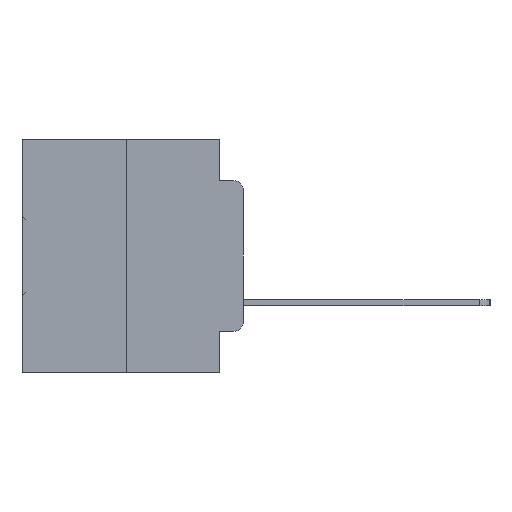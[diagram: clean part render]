
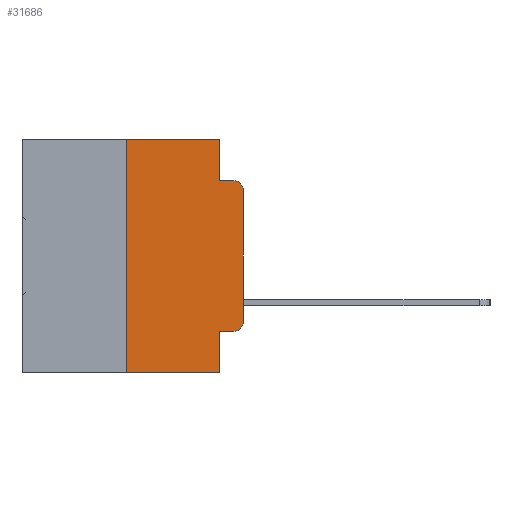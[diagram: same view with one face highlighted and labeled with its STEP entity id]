
A CAD part, left-side view. The second image highlights one B-rep face of the part: STEP entity #31686.
In plain terms, the highlighted planar face has unit normal (-1, 0, 0).
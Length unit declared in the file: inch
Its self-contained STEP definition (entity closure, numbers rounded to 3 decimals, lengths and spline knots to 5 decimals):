
#18 = LINE ( 'NONE', #4390, #19314 ) ;
#545 = CARTESIAN_POINT ( 'NONE',  ( 0., 0.051, -0.0885 ) ) ;
#846 = CARTESIAN_POINT ( 'NONE',  ( 0., 0.02, -0.0885 ) ) ;
#1336 = DIRECTION ( 'NONE',  ( -1., 0., 0. ) ) ;
#1484 = DIRECTION ( 'NONE',  ( 1., 0., 0. ) ) ;
#1604 = VERTEX_POINT ( 'NONE', #846 ) ;
#2535 = VERTEX_POINT ( 'NONE', #27322 ) ;
#2682 = CARTESIAN_POINT ( 'NONE',  ( 0., 0.02, -0.4115 ) ) ;
#3619 = VECTOR ( 'NONE', #10777, 39.37008 ) ;
#3819 = VERTEX_POINT ( 'NONE', #11487 ) ;
#3992 = EDGE_CURVE ( 'NONE', #10135, #1604, #17710, .T. ) ;
#4390 = CARTESIAN_POINT ( 'NONE',  ( 0., 0., 0. ) ) ;
#5689 = EDGE_CURVE ( 'NONE', #13016, #10135, #18, .T. ) ;
#5801 = DIRECTION ( 'NONE',  ( 0., -1., 0. ) ) ;
#5893 = EDGE_CURVE ( 'NONE', #17579, #13016, #7960, .T. ) ;
#6209 = VECTOR ( 'NONE', #22837, 39.37008 ) ;
#6605 = PLANE ( 'NONE',  #25079 ) ;
#7326 = CARTESIAN_POINT ( 'NONE',  ( 0., 0.473, -0.5 ) ) ;
#7960 = CIRCLE ( 'NONE', #10447, 0.02 ) ;
#8567 = EDGE_CURVE ( 'NONE', #21076, #2535, #12137, .T. ) ;
#9147 = DIRECTION ( 'NONE',  ( 0., 0., -1. ) ) ;
#9686 = LINE ( 'NONE', #28645, #22081 ) ;
#10097 = VECTOR ( 'NONE', #10678, 39.37008 ) ;
#10131 = ORIENTED_EDGE ( 'NONE', *, *, #5893, .T. ) ;
#10135 = VERTEX_POINT ( 'NONE', #13831 ) ;
#10249 = DIRECTION ( 'NONE',  ( -1., 0., 0. ) ) ;
#10447 = AXIS2_PLACEMENT_3D ( 'NONE', #24980, #10249, #27399 ) ;
#10678 = DIRECTION ( 'NONE',  ( 0., 0., -1. ) ) ;
#10777 = DIRECTION ( 'NONE',  ( 0., -1., 0. ) ) ;
#10806 = CARTESIAN_POINT ( 'NONE',  ( 0., 0.051, -0.4115 ) ) ;
#11172 = LINE ( 'NONE', #545, #3619 ) ;
#11487 = CARTESIAN_POINT ( 'NONE',  ( 0., 0.051, -0.4115 ) ) ;
#11567 = VECTOR ( 'NONE', #5801, 39.37008 ) ;
#12137 = LINE ( 'NONE', #7326, #13696 ) ;
#12926 = LINE ( 'NONE', #22641, #6209 ) ;
#12977 = EDGE_LOOP ( 'NONE', ( #24627, #15839, #28001, #27245, #19324, #24982, #16242, #21988, #14948, #10131 ) ) ;
#13016 = VERTEX_POINT ( 'NONE', #30482 ) ;
#13696 = VECTOR ( 'NONE', #22214, 39.37008 ) ;
#13732 = EDGE_CURVE ( 'NONE', #21076, #17816, #12926, .T. ) ;
#13831 = CARTESIAN_POINT ( 'NONE',  ( 0., 0., -0.1085 ) ) ;
#14414 = CARTESIAN_POINT ( 'NONE',  ( 0., 0.051, -0.0885 ) ) ;
#14948 = ORIENTED_EDGE ( 'NONE', *, *, #17677, .T. ) ;
#15158 = EDGE_CURVE ( 'NONE', #17816, #30153, #9686, .T. ) ;
#15839 = ORIENTED_EDGE ( 'NONE', *, *, #3992, .T. ) ;
#16242 = ORIENTED_EDGE ( 'NONE', *, *, #8567, .T. ) ;
#16471 = EDGE_CURVE ( 'NONE', #19759, #1604, #11172, .T. ) ;
#16482 = CARTESIAN_POINT ( 'NONE',  ( 0., 0.02, -0.1085 ) ) ;
#17579 = VERTEX_POINT ( 'NONE', #2682 ) ;
#17677 = EDGE_CURVE ( 'NONE', #3819, #17579, #18167, .T. ) ;
#17710 = CIRCLE ( 'NONE', #24645, 0.02 ) ;
#17816 = VERTEX_POINT ( 'NONE', #28445 ) ;
#18167 = LINE ( 'NONE', #10806, #11567 ) ;
#19065 = CARTESIAN_POINT ( 'NONE',  ( 0., 0.473, 0. ) ) ;
#19127 = DIRECTION ( 'NONE',  ( 0., 0., -1. ) ) ;
#19314 = VECTOR ( 'NONE', #28897, 39.37008 ) ;
#19324 = ORIENTED_EDGE ( 'NONE', *, *, #15158, .F. ) ;
#19759 = VERTEX_POINT ( 'NONE', #14414 ) ;
#21076 = VERTEX_POINT ( 'NONE', #22288 ) ;
#21422 = LINE ( 'NONE', #31138, #27053 ) ;
#21988 = ORIENTED_EDGE ( 'NONE', *, *, #27400, .F. ) ;
#22081 = VECTOR ( 'NONE', #31165, 39.37008 ) ;
#22214 = DIRECTION ( 'NONE',  ( 0., -1., 0. ) ) ;
#22288 = CARTESIAN_POINT ( 'NONE',  ( 0., 0.25, -0.5 ) ) ;
#22641 = CARTESIAN_POINT ( 'NONE',  ( 0., 0.25, 0. ) ) ;
#22837 = DIRECTION ( 'NONE',  ( 0., 0., 1. ) ) ;
#23238 = LINE ( 'NONE', #27800, #10097 ) ;
#24627 = ORIENTED_EDGE ( 'NONE', *, *, #5689, .T. ) ;
#24645 = AXIS2_PLACEMENT_3D ( 'NONE', #16482, #1336, #31244 ) ;
#24980 = CARTESIAN_POINT ( 'NONE',  ( 0., 0.02, -0.3915 ) ) ;
#24982 = ORIENTED_EDGE ( 'NONE', *, *, #13732, .F. ) ;
#25079 = AXIS2_PLACEMENT_3D ( 'NONE', #19065, #1484, #9147 ) ;
#27053 = VECTOR ( 'NONE', #19127, 39.37008 ) ;
#27245 = ORIENTED_EDGE ( 'NONE', *, *, #28425, .F. ) ;
#27322 = CARTESIAN_POINT ( 'NONE',  ( 0., 0.051, -0.5 ) ) ;
#27399 = DIRECTION ( 'NONE',  ( 0., 0., -1. ) ) ;
#27400 = EDGE_CURVE ( 'NONE', #3819, #2535, #21422, .T. ) ;
#27466 = CARTESIAN_POINT ( 'NONE',  ( 0., 0.051, 0. ) ) ;
#27800 = CARTESIAN_POINT ( 'NONE',  ( 0., 0.051, 0. ) ) ;
#28001 = ORIENTED_EDGE ( 'NONE', *, *, #16471, .F. ) ;
#28425 = EDGE_CURVE ( 'NONE', #30153, #19759, #23238, .T. ) ;
#28445 = CARTESIAN_POINT ( 'NONE',  ( 0., 0.25, 0. ) ) ;
#28645 = CARTESIAN_POINT ( 'NONE',  ( 0., 0.473, 0. ) ) ;
#28897 = DIRECTION ( 'NONE',  ( 0., 0., 1. ) ) ;
#30153 = VERTEX_POINT ( 'NONE', #27466 ) ;
#30482 = CARTESIAN_POINT ( 'NONE',  ( 0., 0., -0.3915 ) ) ;
#31138 = CARTESIAN_POINT ( 'NONE',  ( 0., 0.051, 0. ) ) ;
#31165 = DIRECTION ( 'NONE',  ( 0., -1., 0. ) ) ;
#31244 = DIRECTION ( 'NONE',  ( 0., 0., -1. ) ) ;
#31282 = FACE_OUTER_BOUND ( 'NONE', #12977, .T. ) ;
#31686 = ADVANCED_FACE ( 'NONE', ( #31282 ), #6605, .F. ) ;
